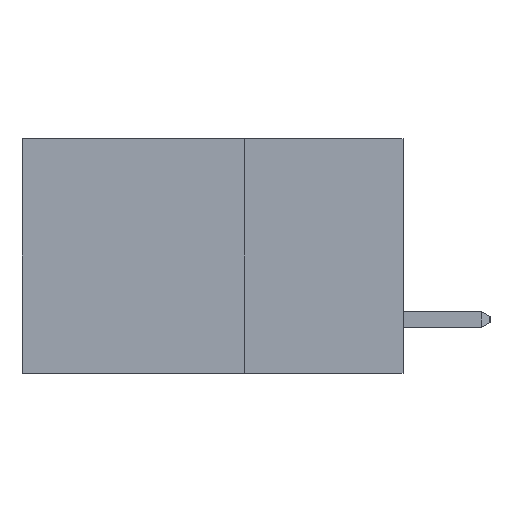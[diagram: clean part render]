
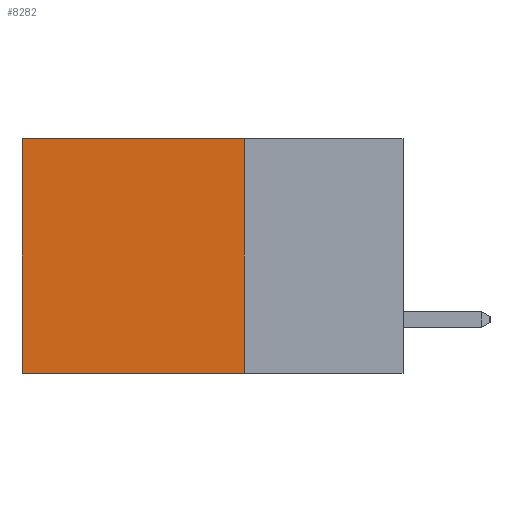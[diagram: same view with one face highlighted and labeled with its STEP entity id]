
A CAD part, left-side view. The second image highlights one B-rep face of the part: STEP entity #8282.
In plain terms, the highlighted planar face has unit normal (-1, 0, 0).
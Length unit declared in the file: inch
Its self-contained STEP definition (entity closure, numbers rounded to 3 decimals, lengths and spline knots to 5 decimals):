
#989 = CARTESIAN_POINT ( 'NONE',  ( 0.2875, 0.6, -0.37 ) ) ;
#1134 = ORIENTED_EDGE ( 'NONE', *, *, #14378, .F. ) ;
#1191 = LINE ( 'NONE', #20410, #20021 ) ;
#1889 = EDGE_LOOP ( 'NONE', ( #10674, #1134, #5236, #18573 ) ) ;
#1980 = FACE_OUTER_BOUND ( 'NONE', #1889, .T. ) ;
#3094 = DIRECTION ( 'NONE',  ( 1., 0., 0. ) ) ;
#3145 = VECTOR ( 'NONE', #17748, 39.37008 ) ;
#3682 = LINE ( 'NONE', #14275, #15341 ) ;
#4515 = EDGE_CURVE ( 'NONE', #14168, #19933, #20505, .T. ) ;
#5236 = ORIENTED_EDGE ( 'NONE', *, *, #4515, .F. ) ;
#6306 = CARTESIAN_POINT ( 'NONE',  ( 0.2875, 0.25, 0. ) ) ;
#6421 = DIRECTION ( 'NONE',  ( 0., 0., -1. ) ) ;
#7866 = AXIS2_PLACEMENT_3D ( 'NONE', #15657, #3094, #10956 ) ;
#7978 = EDGE_CURVE ( 'NONE', #14168, #17739, #15651, .T. ) ;
#8282 = ADVANCED_FACE ( 'NONE', ( #1980 ), #9403, .F. ) ;
#9403 = PLANE ( 'NONE',  #7866 ) ;
#9433 = VECTOR ( 'NONE', #11640, 39.37008 ) ;
#9785 = CARTESIAN_POINT ( 'NONE',  ( 0.2875, 0.25, 0. ) ) ;
#10674 = ORIENTED_EDGE ( 'NONE', *, *, #14872, .T. ) ;
#10956 = DIRECTION ( 'NONE',  ( 0., 0., -1. ) ) ;
#11640 = DIRECTION ( 'NONE',  ( 0., 1., 0. ) ) ;
#14168 = VERTEX_POINT ( 'NONE', #6306 ) ;
#14275 = CARTESIAN_POINT ( 'NONE',  ( 0.2875, 0.25, -0.37 ) ) ;
#14378 = EDGE_CURVE ( 'NONE', #19933, #17188, #3682, .T. ) ;
#14779 = CARTESIAN_POINT ( 'NONE',  ( 0.2875, 0.25, -0.37 ) ) ;
#14872 = EDGE_CURVE ( 'NONE', #17739, #17188, #1191, .T. ) ;
#15341 = VECTOR ( 'NONE', #16123, 39.37008 ) ;
#15651 = LINE ( 'NONE', #16200, #9433 ) ;
#15657 = CARTESIAN_POINT ( 'NONE',  ( 0.2875, 0.25, 0. ) ) ;
#16123 = DIRECTION ( 'NONE',  ( 0., 1., 0. ) ) ;
#16200 = CARTESIAN_POINT ( 'NONE',  ( 0.2875, 0.25, 0. ) ) ;
#17188 = VERTEX_POINT ( 'NONE', #989 ) ;
#17739 = VERTEX_POINT ( 'NONE', #18128 ) ;
#17748 = DIRECTION ( 'NONE',  ( 0., 0., -1. ) ) ;
#18128 = CARTESIAN_POINT ( 'NONE',  ( 0.2875, 0.6, 0. ) ) ;
#18573 = ORIENTED_EDGE ( 'NONE', *, *, #7978, .T. ) ;
#19933 = VERTEX_POINT ( 'NONE', #14779 ) ;
#20021 = VECTOR ( 'NONE', #6421, 39.37008 ) ;
#20410 = CARTESIAN_POINT ( 'NONE',  ( 0.2875, 0.6, 0. ) ) ;
#20505 = LINE ( 'NONE', #9785, #3145 ) ;
